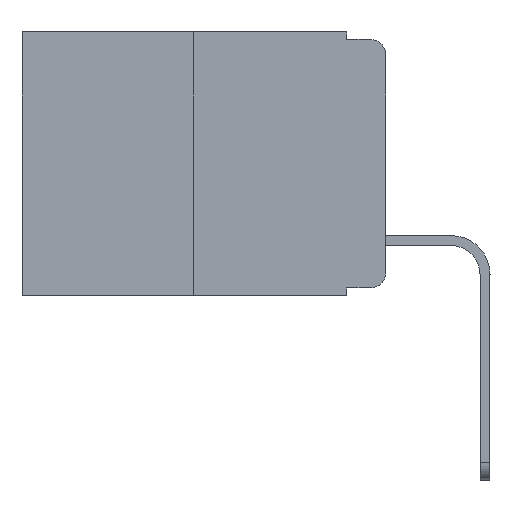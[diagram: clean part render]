
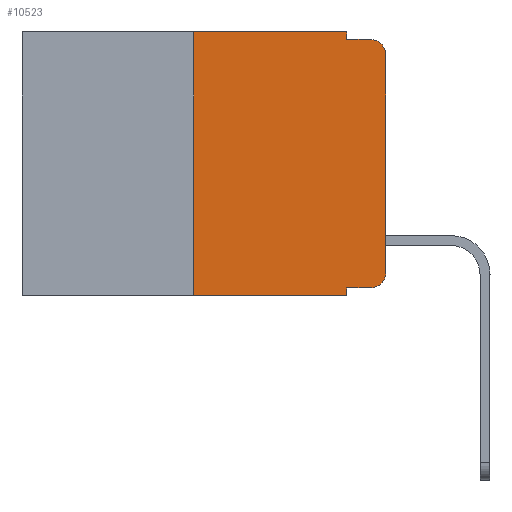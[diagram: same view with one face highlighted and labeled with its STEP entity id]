
A CAD part, left-side view. The second image highlights one B-rep face of the part: STEP entity #10523.
In plain terms, the highlighted planar face has unit normal (-1, 0, 0).
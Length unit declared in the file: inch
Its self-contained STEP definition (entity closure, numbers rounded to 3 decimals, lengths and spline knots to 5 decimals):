
#444 = CARTESIAN_POINT ( 'NONE',  ( 0., 0.051, -0.343 ) ) ;
#690 = VERTEX_POINT ( 'NONE', #8711 ) ;
#965 = CARTESIAN_POINT ( 'NONE',  ( 0., 0.051, 0. ) ) ;
#1112 = ORIENTED_EDGE ( 'NONE', *, *, #3635, .F. ) ;
#1329 = CARTESIAN_POINT ( 'NONE',  ( 0., 0.051, -0.333 ) ) ;
#1612 = VERTEX_POINT ( 'NONE', #444 ) ;
#1653 = CARTESIAN_POINT ( 'NONE',  ( 0., 0.25, 0. ) ) ;
#1676 = DIRECTION ( 'NONE',  ( 0., -1., 0. ) ) ;
#1783 = LINE ( 'NONE', #1329, #4368 ) ;
#2230 = EDGE_LOOP ( 'NONE', ( #15810, #16948, #12972, #1112, #15149, #9770, #15758, #12231, #14363, #6143 ) ) ;
#2350 = VECTOR ( 'NONE', #2787, 39.37008 ) ;
#2470 = EDGE_CURVE ( 'NONE', #13983, #12968, #13991, .T. ) ;
#2760 = CARTESIAN_POINT ( 'NONE',  ( 0., 0.051, -0.01 ) ) ;
#2787 = DIRECTION ( 'NONE',  ( 0., 0., -1. ) ) ;
#3591 = CARTESIAN_POINT ( 'NONE',  ( 0., 0.473, 0. ) ) ;
#3635 = EDGE_CURVE ( 'NONE', #9552, #13983, #18129, .T. ) ;
#3971 = LINE ( 'NONE', #965, #8873 ) ;
#4037 = CARTESIAN_POINT ( 'NONE',  ( 0., 0.473, 0. ) ) ;
#4241 = AXIS2_PLACEMENT_3D ( 'NONE', #3591, #16918, #18469 ) ;
#4342 = DIRECTION ( 'NONE',  ( 0., 0., -1. ) ) ;
#4368 = VECTOR ( 'NONE', #11682, 39.37008 ) ;
#5006 = CARTESIAN_POINT ( 'NONE',  ( 0., 0.051, -0.01 ) ) ;
#5122 = EDGE_CURVE ( 'NONE', #13735, #690, #9615, .T. ) ;
#5991 = VERTEX_POINT ( 'NONE', #16415 ) ;
#6143 = ORIENTED_EDGE ( 'NONE', *, *, #18336, .T. ) ;
#6303 = DIRECTION ( 'NONE',  ( 0., -1., 0. ) ) ;
#6733 = CARTESIAN_POINT ( 'NONE',  ( 0., 0.02, -0.01 ) ) ;
#6760 = FACE_OUTER_BOUND ( 'NONE', #2230, .T. ) ;
#6795 = AXIS2_PLACEMENT_3D ( 'NONE', #10241, #10116, #4342 ) ;
#6833 = EDGE_CURVE ( 'NONE', #5991, #1612, #3971, .T. ) ;
#6894 = DIRECTION ( 'NONE',  ( 0., -1., 0. ) ) ;
#7070 = CARTESIAN_POINT ( 'NONE',  ( 0., 0.051, 0. ) ) ;
#7413 = AXIS2_PLACEMENT_3D ( 'NONE', #16808, #12216, #16682 ) ;
#7649 = CARTESIAN_POINT ( 'NONE',  ( 0., 0.25, -0.343 ) ) ;
#8343 = CIRCLE ( 'NONE', #7413, 0.02 ) ;
#8502 = EDGE_CURVE ( 'NONE', #5991, #9579, #1783, .T. ) ;
#8664 = CARTESIAN_POINT ( 'NONE',  ( 0., 0.051, 0. ) ) ;
#8711 = CARTESIAN_POINT ( 'NONE',  ( 0., 0., -0.03 ) ) ;
#8873 = VECTOR ( 'NONE', #12738, 39.37008 ) ;
#9552 = VERTEX_POINT ( 'NONE', #7070 ) ;
#9579 = VERTEX_POINT ( 'NONE', #15717 ) ;
#9615 = LINE ( 'NONE', #14480, #17674 ) ;
#9770 = ORIENTED_EDGE ( 'NONE', *, *, #18447, .F. ) ;
#9891 = CARTESIAN_POINT ( 'NONE',  ( 0., 0.25, 0. ) ) ;
#10026 = LINE ( 'NONE', #4037, #10268 ) ;
#10116 = DIRECTION ( 'NONE',  ( -1., 0., 0. ) ) ;
#10241 = CARTESIAN_POINT ( 'NONE',  ( 0., 0.02, -0.313 ) ) ;
#10268 = VECTOR ( 'NONE', #6894, 39.37008 ) ;
#10523 = ADVANCED_FACE ( 'NONE', ( #6760 ), #12458, .F. ) ;
#10663 = EDGE_CURVE ( 'NONE', #13253, #9552, #10026, .T. ) ;
#11210 = VECTOR ( 'NONE', #6303, 39.37008 ) ;
#11682 = DIRECTION ( 'NONE',  ( 0., -1., 0. ) ) ;
#12216 = DIRECTION ( 'NONE',  ( -1., 0., 0. ) ) ;
#12231 = ORIENTED_EDGE ( 'NONE', *, *, #6833, .F. ) ;
#12458 = PLANE ( 'NONE',  #4241 ) ;
#12496 = CARTESIAN_POINT ( 'NONE',  ( 0., 0., -0.313 ) ) ;
#12738 = DIRECTION ( 'NONE',  ( 0., 0., -1. ) ) ;
#12968 = VERTEX_POINT ( 'NONE', #6733 ) ;
#12972 = ORIENTED_EDGE ( 'NONE', *, *, #2470, .F. ) ;
#13253 = VERTEX_POINT ( 'NONE', #9891 ) ;
#13735 = VERTEX_POINT ( 'NONE', #12496 ) ;
#13983 = VERTEX_POINT ( 'NONE', #2760 ) ;
#13991 = LINE ( 'NONE', #5006, #11210 ) ;
#14133 = VERTEX_POINT ( 'NONE', #7649 ) ;
#14289 = CIRCLE ( 'NONE', #6795, 0.02 ) ;
#14363 = ORIENTED_EDGE ( 'NONE', *, *, #8502, .T. ) ;
#14480 = CARTESIAN_POINT ( 'NONE',  ( 0., 0., 0. ) ) ;
#14935 = CARTESIAN_POINT ( 'NONE',  ( 0., 0.473, -0.343 ) ) ;
#14979 = DIRECTION ( 'NONE',  ( 0., 0., 1. ) ) ;
#15149 = ORIENTED_EDGE ( 'NONE', *, *, #10663, .F. ) ;
#15717 = CARTESIAN_POINT ( 'NONE',  ( 0., 0.02, -0.333 ) ) ;
#15758 = ORIENTED_EDGE ( 'NONE', *, *, #19083, .T. ) ;
#15810 = ORIENTED_EDGE ( 'NONE', *, *, #5122, .T. ) ;
#16415 = CARTESIAN_POINT ( 'NONE',  ( 0., 0.051, -0.333 ) ) ;
#16682 = DIRECTION ( 'NONE',  ( 0., 0., -1. ) ) ;
#16808 = CARTESIAN_POINT ( 'NONE',  ( 0., 0.02, -0.03 ) ) ;
#16864 = EDGE_CURVE ( 'NONE', #690, #12968, #8343, .T. ) ;
#16918 = DIRECTION ( 'NONE',  ( 1., 0., 0. ) ) ;
#16948 = ORIENTED_EDGE ( 'NONE', *, *, #16864, .T. ) ;
#17065 = VECTOR ( 'NONE', #1676, 39.37008 ) ;
#17279 = DIRECTION ( 'NONE',  ( 0., 0., 1. ) ) ;
#17522 = LINE ( 'NONE', #14935, #17065 ) ;
#17674 = VECTOR ( 'NONE', #17279, 39.37008 ) ;
#17790 = VECTOR ( 'NONE', #14979, 39.37008 ) ;
#18129 = LINE ( 'NONE', #8664, #2350 ) ;
#18248 = LINE ( 'NONE', #1653, #17790 ) ;
#18336 = EDGE_CURVE ( 'NONE', #9579, #13735, #14289, .T. ) ;
#18447 = EDGE_CURVE ( 'NONE', #14133, #13253, #18248, .T. ) ;
#18469 = DIRECTION ( 'NONE',  ( 0., 0., -1. ) ) ;
#19083 = EDGE_CURVE ( 'NONE', #14133, #1612, #17522, .T. ) ;
